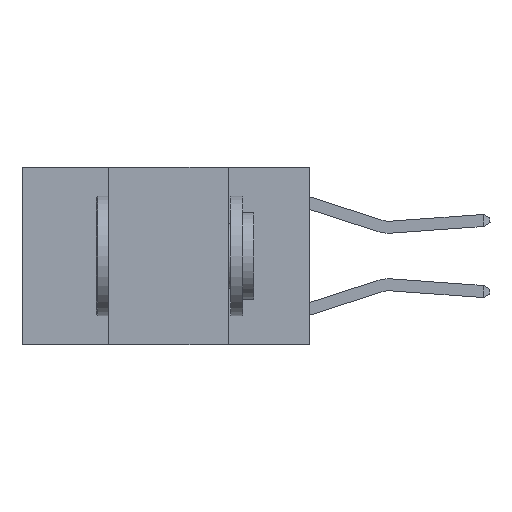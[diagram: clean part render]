
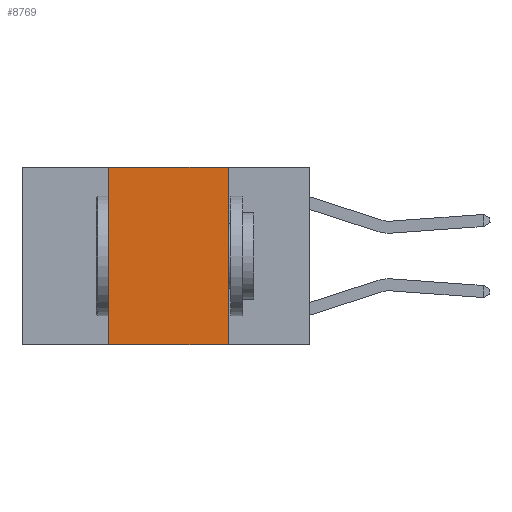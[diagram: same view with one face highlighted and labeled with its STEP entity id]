
A CAD part, left-side view. The second image highlights one B-rep face of the part: STEP entity #8769.
In plain terms, the highlighted planar face has unit normal (-1, 0, 0).
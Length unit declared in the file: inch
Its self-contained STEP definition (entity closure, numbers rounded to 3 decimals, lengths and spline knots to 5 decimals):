
#951 = LINE ( 'NONE', #8027, #5936 ) ;
#1219 = DIRECTION ( 'NONE',  ( 1., 0., 0. ) ) ;
#1258 = CARTESIAN_POINT ( 'NONE',  ( 0., 0.6, -0.37 ) ) ;
#1295 = DIRECTION ( 'NONE',  ( 0., 0., -1. ) ) ;
#1331 = CARTESIAN_POINT ( 'NONE',  ( 0., 0.17, 0. ) ) ;
#2840 = ORIENTED_EDGE ( 'NONE', *, *, #2945, .F. ) ;
#2945 = EDGE_CURVE ( 'NONE', #7406, #8168, #6521, .T. ) ;
#3029 = ORIENTED_EDGE ( 'NONE', *, *, #5636, .F. ) ;
#3063 = ORIENTED_EDGE ( 'NONE', *, *, #3705, .F. ) ;
#3139 = ORIENTED_EDGE ( 'NONE', *, *, #3835, .T. ) ;
#3159 = CARTESIAN_POINT ( 'NONE',  ( 0., 0.17, 0. ) ) ;
#3668 = VECTOR ( 'NONE', #9660, 39.37008 ) ;
#3705 = EDGE_CURVE ( 'NONE', #7646, #8730, #5825, .T. ) ;
#3835 = EDGE_CURVE ( 'NONE', #7646, #8168, #8837, .T. ) ;
#3887 = CARTESIAN_POINT ( 'NONE',  ( 0., 0.42, 0. ) ) ;
#4714 = VECTOR ( 'NONE', #1295, 39.37008 ) ;
#5351 = AXIS2_PLACEMENT_3D ( 'NONE', #9039, #1219, #7575 ) ;
#5636 = EDGE_CURVE ( 'NONE', #8730, #7406, #951, .T. ) ;
#5825 = LINE ( 'NONE', #3887, #3668 ) ;
#5936 = VECTOR ( 'NONE', #10904, 39.37008 ) ;
#6396 = CARTESIAN_POINT ( 'NONE',  ( 0., 0.17, -0.37 ) ) ;
#6493 = VECTOR ( 'NONE', #9814, 39.37008 ) ;
#6521 = LINE ( 'NONE', #3159, #4714 ) ;
#6739 = PLANE ( 'NONE',  #5351 ) ;
#7406 = VERTEX_POINT ( 'NONE', #1331 ) ;
#7575 = DIRECTION ( 'NONE',  ( 0., 0., -1. ) ) ;
#7646 = VERTEX_POINT ( 'NONE', #9993 ) ;
#8027 = CARTESIAN_POINT ( 'NONE',  ( 0., 0.6, 0. ) ) ;
#8168 = VERTEX_POINT ( 'NONE', #6396 ) ;
#8730 = VERTEX_POINT ( 'NONE', #9756 ) ;
#8769 = ADVANCED_FACE ( 'NONE', ( #10126 ), #6739, .F. ) ;
#8837 = LINE ( 'NONE', #1258, #6493 ) ;
#9039 = CARTESIAN_POINT ( 'NONE',  ( 0., 0.6, 0. ) ) ;
#9405 = EDGE_LOOP ( 'NONE', ( #2840, #3029, #3063, #3139 ) ) ;
#9660 = DIRECTION ( 'NONE',  ( 0., 0., 1. ) ) ;
#9756 = CARTESIAN_POINT ( 'NONE',  ( 0., 0.42, 0. ) ) ;
#9814 = DIRECTION ( 'NONE',  ( 0., -1., 0. ) ) ;
#9993 = CARTESIAN_POINT ( 'NONE',  ( 0., 0.42, -0.37 ) ) ;
#10126 = FACE_OUTER_BOUND ( 'NONE', #9405, .T. ) ;
#10904 = DIRECTION ( 'NONE',  ( 0., -1., 0. ) ) ;
